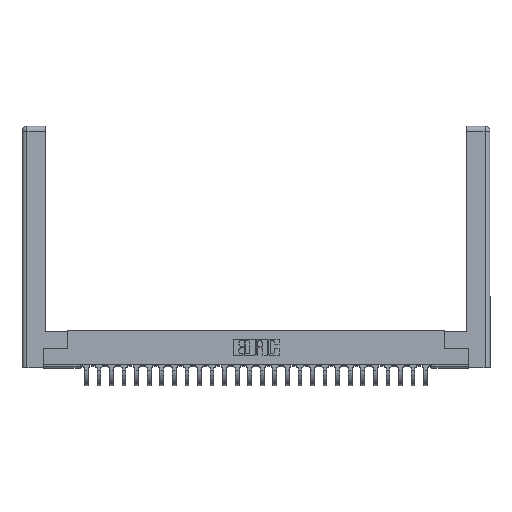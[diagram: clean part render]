
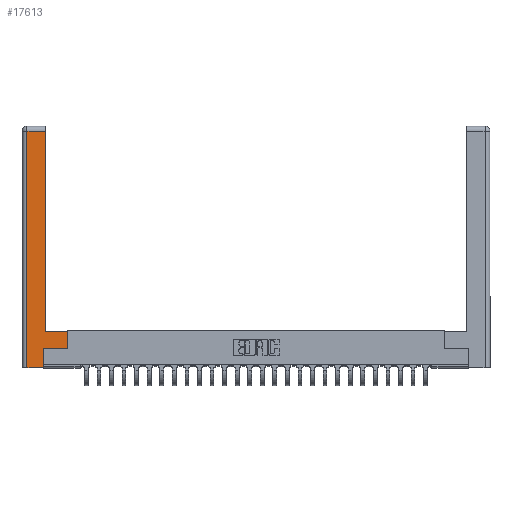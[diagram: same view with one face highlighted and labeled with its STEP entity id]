
A CAD part, top view. The second image highlights one B-rep face of the part: STEP entity #17613.
In plain terms, the highlighted planar face has unit normal (0, 0, 1).
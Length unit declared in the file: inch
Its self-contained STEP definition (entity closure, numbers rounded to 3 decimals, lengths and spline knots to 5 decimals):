
#746 = CARTESIAN_POINT ( 'NONE',  ( 0.295, 0.45, 0. ) ) ;
#1512 = VECTOR ( 'NONE', #6564, 39.37008 ) ;
#2592 = CARTESIAN_POINT ( 'NONE',  ( 0.265, 0.245, 0. ) ) ;
#2845 = CARTESIAN_POINT ( 'NONE',  ( 0.565, 0.245, 0. ) ) ;
#2942 = CARTESIAN_POINT ( 'NONE',  ( 0.265, 0., 0. ) ) ;
#3150 = LINE ( 'NONE', #2845, #5187 ) ;
#4543 = DIRECTION ( 'NONE',  ( 1., 0., 0. ) ) ;
#4997 = CARTESIAN_POINT ( 'NONE',  ( 0.265, 0., 0. ) ) ;
#5045 = EDGE_CURVE ( 'NONE', #12227, #24429, #11862, .T. ) ;
#5187 = VECTOR ( 'NONE', #21816, 39.37008 ) ;
#5307 = CARTESIAN_POINT ( 'NONE',  ( 0.0615, 0., 0. ) ) ;
#5314 = ORIENTED_EDGE ( 'NONE', *, *, #27736, .T. ) ;
#5608 = ORIENTED_EDGE ( 'NONE', *, *, #26683, .T. ) ;
#6341 = EDGE_LOOP ( 'NONE', ( #5608, #15912, #29674, #10754, #5314, #27007, #11850, #25550 ) ) ;
#6564 = DIRECTION ( 'NONE',  ( -1., 0., 0. ) ) ;
#8211 = VECTOR ( 'NONE', #13658, 39.37008 ) ;
#8612 = CARTESIAN_POINT ( 'NONE',  ( 0.295, 3., 0. ) ) ;
#10736 = CARTESIAN_POINT ( 'NONE',  ( 0.265, 0.245, 0. ) ) ;
#10754 = ORIENTED_EDGE ( 'NONE', *, *, #5045, .T. ) ;
#11096 = VECTOR ( 'NONE', #4543, 39.37008 ) ;
#11719 = LINE ( 'NONE', #18553, #1512 ) ;
#11724 = EDGE_CURVE ( 'NONE', #15555, #12227, #15680, .T. ) ;
#11850 = ORIENTED_EDGE ( 'NONE', *, *, #21560, .T. ) ;
#11862 = LINE ( 'NONE', #4997, #11096 ) ;
#11950 = AXIS2_PLACEMENT_3D ( 'NONE', #28779, #23946, #23663 ) ;
#12110 = EDGE_CURVE ( 'NONE', #17281, #18654, #11719, .T. ) ;
#12227 = VERTEX_POINT ( 'NONE', #5307 ) ;
#12555 = DIRECTION ( 'NONE',  ( 0., 1., 0. ) ) ;
#13422 = LINE ( 'NONE', #8612, #21006 ) ;
#13601 = EDGE_CURVE ( 'NONE', #29433, #15555, #25468, .T. ) ;
#13658 = DIRECTION ( 'NONE',  ( 0., -1., 0. ) ) ;
#13814 = CARTESIAN_POINT ( 'NONE',  ( 0.0615, 2.94, 0. ) ) ;
#14425 = VERTEX_POINT ( 'NONE', #26135 ) ;
#14433 = LINE ( 'NONE', #2592, #24022 ) ;
#15555 = VERTEX_POINT ( 'NONE', #24932 ) ;
#15560 = LINE ( 'NONE', #25045, #29067 ) ;
#15680 = LINE ( 'NONE', #23139, #8211 ) ;
#15912 = ORIENTED_EDGE ( 'NONE', *, *, #13601, .T. ) ;
#17157 = CARTESIAN_POINT ( 'NONE',  ( 0.565, 0.45, 0. ) ) ;
#17281 = VERTEX_POINT ( 'NONE', #17157 ) ;
#17613 = ADVANCED_FACE ( 'NONE', ( #26428 ), #19283, .F. ) ;
#18553 = CARTESIAN_POINT ( 'NONE',  ( 0.295, 0.45, 0. ) ) ;
#18654 = VERTEX_POINT ( 'NONE', #746 ) ;
#19283 = PLANE ( 'NONE',  #11950 ) ;
#20969 = EDGE_CURVE ( 'NONE', #28811, #14425, #3150, .T. ) ;
#21006 = VECTOR ( 'NONE', #25391, 39.37008 ) ;
#21560 = EDGE_CURVE ( 'NONE', #14425, #17281, #15560, .T. ) ;
#21816 = DIRECTION ( 'NONE',  ( 1., 0., 0. ) ) ;
#22709 = DIRECTION ( 'NONE',  ( 0., 1., 0. ) ) ;
#23139 = CARTESIAN_POINT ( 'NONE',  ( 0.0615, 0., 0. ) ) ;
#23149 = DIRECTION ( 'NONE',  ( -1., 0., 0. ) ) ;
#23663 = DIRECTION ( 'NONE',  ( -1., 0., 0. ) ) ;
#23946 = DIRECTION ( 'NONE',  ( 0., 0., -1. ) ) ;
#24022 = VECTOR ( 'NONE', #12555, 39.37008 ) ;
#24429 = VERTEX_POINT ( 'NONE', #2942 ) ;
#24932 = CARTESIAN_POINT ( 'NONE',  ( 0.0615, 2.94, 0. ) ) ;
#25045 = CARTESIAN_POINT ( 'NONE',  ( 0.565, 0.45, 0. ) ) ;
#25391 = DIRECTION ( 'NONE',  ( 0., 1., 0. ) ) ;
#25468 = LINE ( 'NONE', #13814, #26910 ) ;
#25550 = ORIENTED_EDGE ( 'NONE', *, *, #12110, .T. ) ;
#26135 = CARTESIAN_POINT ( 'NONE',  ( 0.565, 0.245, 0. ) ) ;
#26428 = FACE_OUTER_BOUND ( 'NONE', #6341, .T. ) ;
#26683 = EDGE_CURVE ( 'NONE', #18654, #29433, #13422, .T. ) ;
#26910 = VECTOR ( 'NONE', #23149, 39.37008 ) ;
#27007 = ORIENTED_EDGE ( 'NONE', *, *, #20969, .T. ) ;
#27736 = EDGE_CURVE ( 'NONE', #24429, #28811, #14433, .T. ) ;
#28103 = CARTESIAN_POINT ( 'NONE',  ( 0.295, 2.94, 0. ) ) ;
#28779 = CARTESIAN_POINT ( 'NONE',  ( 0., 0., 0. ) ) ;
#28811 = VERTEX_POINT ( 'NONE', #10736 ) ;
#29067 = VECTOR ( 'NONE', #22709, 39.37008 ) ;
#29433 = VERTEX_POINT ( 'NONE', #28103 ) ;
#29674 = ORIENTED_EDGE ( 'NONE', *, *, #11724, .T. ) ;
